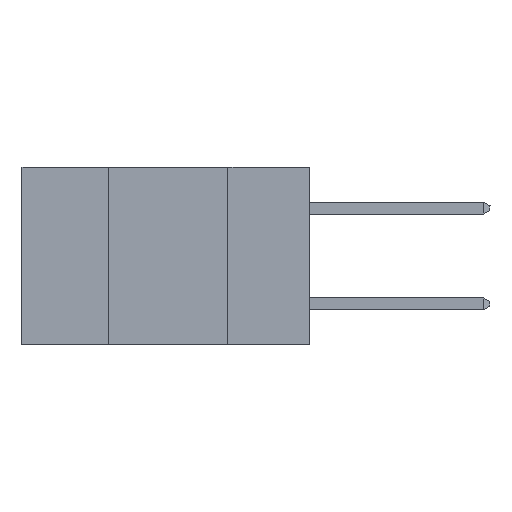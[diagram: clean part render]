
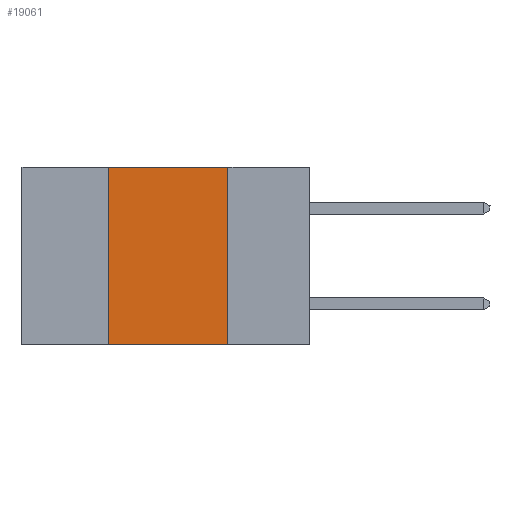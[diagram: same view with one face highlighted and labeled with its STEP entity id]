
A CAD part, left-side view. The second image highlights one B-rep face of the part: STEP entity #19061.
In plain terms, the highlighted planar face has unit normal (-1, 0, 0).
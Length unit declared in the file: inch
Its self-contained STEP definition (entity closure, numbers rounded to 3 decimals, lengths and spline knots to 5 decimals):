
#465 = VERTEX_POINT ( 'NONE', #1665 ) ;
#1665 = CARTESIAN_POINT ( 'NONE',  ( 0., 0.42, 0. ) ) ;
#2152 = DIRECTION ( 'NONE',  ( 0., 0., 1. ) ) ;
#3073 = DIRECTION ( 'NONE',  ( 0., 0., -1. ) ) ;
#3123 = CARTESIAN_POINT ( 'NONE',  ( 0., 0.6, 0. ) ) ;
#3518 = LINE ( 'NONE', #10914, #10986 ) ;
#4706 = LINE ( 'NONE', #16498, #6572 ) ;
#4736 = FACE_OUTER_BOUND ( 'NONE', #15022, .T. ) ;
#4825 = ORIENTED_EDGE ( 'NONE', *, *, #7989, .F. ) ;
#6572 = VECTOR ( 'NONE', #10445, 39.37008 ) ;
#6773 = AXIS2_PLACEMENT_3D ( 'NONE', #16429, #8905, #3073 ) ;
#7592 = DIRECTION ( 'NONE',  ( 0., -1., 0. ) ) ;
#7740 = LINE ( 'NONE', #10475, #17842 ) ;
#7807 = VERTEX_POINT ( 'NONE', #8304 ) ;
#7989 = EDGE_CURVE ( 'NONE', #14470, #12824, #4706, .T. ) ;
#8304 = CARTESIAN_POINT ( 'NONE',  ( 0., 0.42, -0.37 ) ) ;
#8905 = DIRECTION ( 'NONE',  ( 1., 0., 0. ) ) ;
#9838 = CARTESIAN_POINT ( 'NONE',  ( 0., 0.17, -0.37 ) ) ;
#9885 = ORIENTED_EDGE ( 'NONE', *, *, #11720, .F. ) ;
#9887 = EDGE_CURVE ( 'NONE', #7807, #465, #3518, .T. ) ;
#10445 = DIRECTION ( 'NONE',  ( 0., 0., -1. ) ) ;
#10470 = PLANE ( 'NONE',  #6773 ) ;
#10475 = CARTESIAN_POINT ( 'NONE',  ( 0., 0.6, -0.37 ) ) ;
#10852 = EDGE_CURVE ( 'NONE', #7807, #12824, #7740, .T. ) ;
#10867 = DIRECTION ( 'NONE',  ( 0., -1., 0. ) ) ;
#10901 = CARTESIAN_POINT ( 'NONE',  ( 0., 0.17, 0. ) ) ;
#10914 = CARTESIAN_POINT ( 'NONE',  ( 0., 0.42, 0. ) ) ;
#10949 = ORIENTED_EDGE ( 'NONE', *, *, #9887, .F. ) ;
#10986 = VECTOR ( 'NONE', #2152, 39.37008 ) ;
#11720 = EDGE_CURVE ( 'NONE', #465, #14470, #15482, .T. ) ;
#12824 = VERTEX_POINT ( 'NONE', #9838 ) ;
#14248 = ORIENTED_EDGE ( 'NONE', *, *, #10852, .T. ) ;
#14470 = VERTEX_POINT ( 'NONE', #10901 ) ;
#15022 = EDGE_LOOP ( 'NONE', ( #4825, #9885, #10949, #14248 ) ) ;
#15482 = LINE ( 'NONE', #3123, #15719 ) ;
#15719 = VECTOR ( 'NONE', #7592, 39.37008 ) ;
#16429 = CARTESIAN_POINT ( 'NONE',  ( 0., 0.6, 0. ) ) ;
#16498 = CARTESIAN_POINT ( 'NONE',  ( 0., 0.17, 0. ) ) ;
#17842 = VECTOR ( 'NONE', #10867, 39.37008 ) ;
#19061 = ADVANCED_FACE ( 'NONE', ( #4736 ), #10470, .F. ) ;
